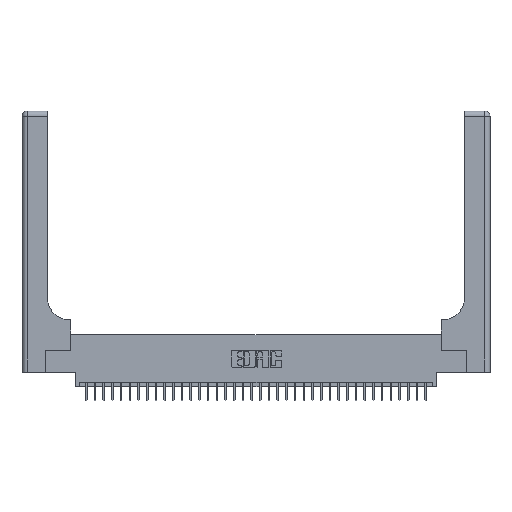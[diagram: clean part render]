
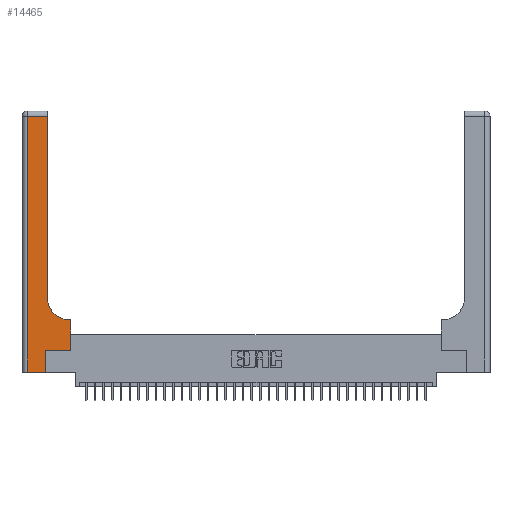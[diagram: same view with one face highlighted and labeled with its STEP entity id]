
A CAD part, top view. The second image highlights one B-rep face of the part: STEP entity #14465.
In plain terms, the highlighted planar face has unit normal (0, 0, 1).
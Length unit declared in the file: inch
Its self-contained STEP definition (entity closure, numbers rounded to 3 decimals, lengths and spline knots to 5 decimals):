
#37 = ORIENTED_EDGE ( 'NONE', *, *, #2687, .T. ) ;
#1096 = AXIS2_PLACEMENT_3D ( 'NONE', #36816, #17039, #17376 ) ;
#1156 = CARTESIAN_POINT ( 'NONE',  ( 0.5585, 0.6, 0.37 ) ) ;
#1357 = VERTEX_POINT ( 'NONE', #28327 ) ;
#2031 = EDGE_CURVE ( 'NONE', #33853, #33589, #10858, .T. ) ;
#2332 = CARTESIAN_POINT ( 'NONE',  ( 0.269, 0.25, 0.37 ) ) ;
#2550 = CARTESIAN_POINT ( 'NONE',  ( 0.06, 0., 0.37 ) ) ;
#2687 = EDGE_CURVE ( 'NONE', #16504, #14867, #4034, .T. ) ;
#2833 = LINE ( 'NONE', #26582, #32287 ) ;
#2862 = EDGE_CURVE ( 'NONE', #1357, #28328, #34467, .T. ) ;
#4034 = LINE ( 'NONE', #26210, #26854 ) ;
#5739 = DIRECTION ( 'NONE',  ( 0., 1., 0. ) ) ;
#6024 = CARTESIAN_POINT ( 'NONE',  ( 0., 2.94, 0.37 ) ) ;
#6077 = VECTOR ( 'NONE', #28092, 39.37008 ) ;
#6106 = EDGE_CURVE ( 'NONE', #7385, #1357, #27678, .T. ) ;
#6250 = DIRECTION ( 'NONE',  ( 1., 0., 0. ) ) ;
#7385 = VERTEX_POINT ( 'NONE', #35688 ) ;
#9015 = EDGE_CURVE ( 'NONE', #23725, #36089, #27499, .T. ) ;
#9211 = ORIENTED_EDGE ( 'NONE', *, *, #24525, .T. ) ;
#10137 = FACE_OUTER_BOUND ( 'NONE', #15391, .T. ) ;
#10762 = CARTESIAN_POINT ( 'NONE',  ( 0.2915, 3., 0.37 ) ) ;
#10858 = LINE ( 'NONE', #33437, #32711 ) ;
#12392 = ORIENTED_EDGE ( 'NONE', *, *, #2031, .T. ) ;
#14465 = ADVANCED_FACE ( 'NONE', ( #10137 ), #33082, .F. ) ;
#14758 = ORIENTED_EDGE ( 'NONE', *, *, #31810, .T. ) ;
#14867 = VERTEX_POINT ( 'NONE', #1156 ) ;
#15012 = ORIENTED_EDGE ( 'NONE', *, *, #9015, .T. ) ;
#15391 = EDGE_LOOP ( 'NONE', ( #20872, #9211, #12392, #17832, #15012, #14758, #37, #31741, #23660 ) ) ;
#16007 = DIRECTION ( 'NONE',  ( 0., 1., 0. ) ) ;
#16504 = VERTEX_POINT ( 'NONE', #24209 ) ;
#17039 = DIRECTION ( 'NONE',  ( 0., 0., -1. ) ) ;
#17281 = DIRECTION ( 'NONE',  ( -1., 0., 0. ) ) ;
#17376 = DIRECTION ( 'NONE',  ( 1., 0., 0. ) ) ;
#17832 = ORIENTED_EDGE ( 'NONE', *, *, #24736, .T. ) ;
#18151 = CARTESIAN_POINT ( 'NONE',  ( 0., 3., 0.37 ) ) ;
#18479 = CARTESIAN_POINT ( 'NONE',  ( 0.269, 0., 0.37 ) ) ;
#19847 = CARTESIAN_POINT ( 'NONE',  ( 0.269, 0., 0.37 ) ) ;
#19919 = VECTOR ( 'NONE', #16007, 39.37008 ) ;
#20314 = VECTOR ( 'NONE', #21803, 39.37008 ) ;
#20872 = ORIENTED_EDGE ( 'NONE', *, *, #2862, .T. ) ;
#21167 = DIRECTION ( 'NONE',  ( -1., 0., 0. ) ) ;
#21803 = DIRECTION ( 'NONE',  ( -1., 0., 0. ) ) ;
#22894 = AXIS2_PLACEMENT_3D ( 'NONE', #18151, #30086, #21167 ) ;
#23299 = CARTESIAN_POINT ( 'NONE',  ( 0.2915, 2.94, 0.37 ) ) ;
#23456 = LINE ( 'NONE', #2332, #6077 ) ;
#23660 = ORIENTED_EDGE ( 'NONE', *, *, #6106, .T. ) ;
#23725 = VERTEX_POINT ( 'NONE', #19847 ) ;
#24209 = CARTESIAN_POINT ( 'NONE',  ( 0.5585, 0.25, 0.37 ) ) ;
#24525 = EDGE_CURVE ( 'NONE', #28328, #33853, #32718, .T. ) ;
#24736 = EDGE_CURVE ( 'NONE', #33589, #23725, #2833, .T. ) ;
#25200 = VECTOR ( 'NONE', #17281, 39.37008 ) ;
#26138 = DIRECTION ( 'NONE',  ( 0., -1., 0. ) ) ;
#26210 = CARTESIAN_POINT ( 'NONE',  ( 0.5585, 0.25, 0.37 ) ) ;
#26582 = CARTESIAN_POINT ( 'NONE',  ( 0., 0., 0.37 ) ) ;
#26854 = VECTOR ( 'NONE', #31976, 39.37008 ) ;
#27314 = CARTESIAN_POINT ( 'NONE',  ( 0.269, 0.25, 0.37 ) ) ;
#27499 = LINE ( 'NONE', #18479, #19919 ) ;
#27678 = CIRCLE ( 'NONE', #1096, 0.25 ) ;
#27937 = LINE ( 'NONE', #27949, #20314 ) ;
#27949 = CARTESIAN_POINT ( 'NONE',  ( 0.2915, 0.6, 0.37 ) ) ;
#28092 = DIRECTION ( 'NONE',  ( 1., 0., 0. ) ) ;
#28327 = CARTESIAN_POINT ( 'NONE',  ( 0.2915, 0.85, 0.37 ) ) ;
#28328 = VERTEX_POINT ( 'NONE', #23299 ) ;
#28991 = CARTESIAN_POINT ( 'NONE',  ( 0.06, 2.94, 0.37 ) ) ;
#30086 = DIRECTION ( 'NONE',  ( 0., 0., -1. ) ) ;
#31741 = ORIENTED_EDGE ( 'NONE', *, *, #32941, .T. ) ;
#31810 = EDGE_CURVE ( 'NONE', #36089, #16504, #23456, .T. ) ;
#31976 = DIRECTION ( 'NONE',  ( 0., 1., 0. ) ) ;
#32287 = VECTOR ( 'NONE', #6250, 39.37008 ) ;
#32711 = VECTOR ( 'NONE', #26138, 39.37008 ) ;
#32718 = LINE ( 'NONE', #6024, #25200 ) ;
#32941 = EDGE_CURVE ( 'NONE', #14867, #7385, #27937, .T. ) ;
#33082 = PLANE ( 'NONE',  #22894 ) ;
#33437 = CARTESIAN_POINT ( 'NONE',  ( 0.06, 3., 0.37 ) ) ;
#33589 = VERTEX_POINT ( 'NONE', #2550 ) ;
#33596 = VECTOR ( 'NONE', #5739, 39.37008 ) ;
#33853 = VERTEX_POINT ( 'NONE', #28991 ) ;
#34467 = LINE ( 'NONE', #10762, #33596 ) ;
#35688 = CARTESIAN_POINT ( 'NONE',  ( 0.5415, 0.6, 0.37 ) ) ;
#36089 = VERTEX_POINT ( 'NONE', #27314 ) ;
#36816 = CARTESIAN_POINT ( 'NONE',  ( 0.5415, 0.85, 0.37 ) ) ;
